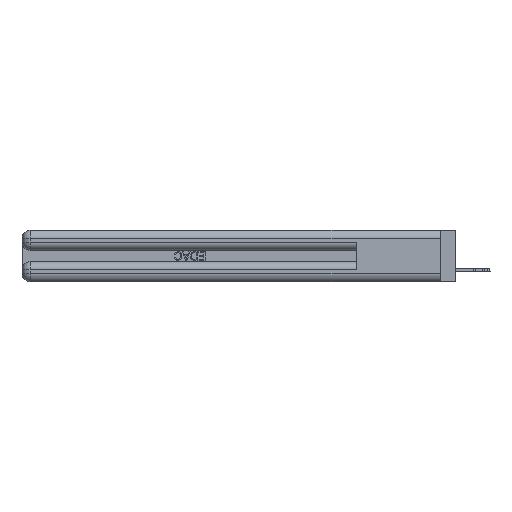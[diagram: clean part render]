
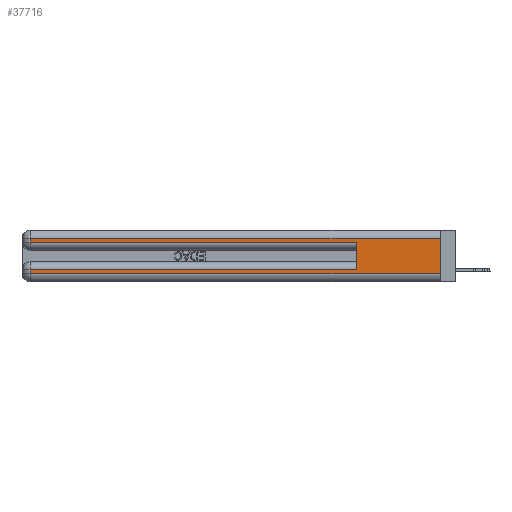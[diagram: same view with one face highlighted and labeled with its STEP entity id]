
A CAD part, left-side view. The second image highlights one B-rep face of the part: STEP entity #37716.
In plain terms, the highlighted planar face has unit normal (-1, 0, 0).
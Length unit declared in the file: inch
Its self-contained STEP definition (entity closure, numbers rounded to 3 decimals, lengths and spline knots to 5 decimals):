
#146 = ORIENTED_EDGE ( 'NONE', *, *, #33059, .T. ) ;
#435 = LINE ( 'NONE', #4650, #18090 ) ;
#865 = VECTOR ( 'NONE', #20401, 39.37008 ) ;
#1054 = FACE_OUTER_BOUND ( 'NONE', #14440, .T. ) ;
#1410 = VECTOR ( 'NONE', #2643, 39.37008 ) ;
#2643 = DIRECTION ( 'NONE',  ( 0., -1., 0. ) ) ;
#2742 = CARTESIAN_POINT ( 'NONE',  ( 0., 2.94, 0.37 ) ) ;
#2978 = EDGE_CURVE ( 'NONE', #9925, #3714, #24033, .T. ) ;
#3238 = LINE ( 'NONE', #29658, #37325 ) ;
#3714 = VERTEX_POINT ( 'NONE', #30575 ) ;
#3871 = VERTEX_POINT ( 'NONE', #29867 ) ;
#4545 = DIRECTION ( 'NONE',  ( 0., 0., -1. ) ) ;
#4615 = ORIENTED_EDGE ( 'NONE', *, *, #8156, .T. ) ;
#4650 = CARTESIAN_POINT ( 'NONE',  ( 0., 2.94, 0.37 ) ) ;
#4687 = CARTESIAN_POINT ( 'NONE',  ( 0., 0., 0.37 ) ) ;
#6514 = LINE ( 'NONE', #2742, #865 ) ;
#7656 = DIRECTION ( 'NONE',  ( 1., 0., 0. ) ) ;
#8156 = EDGE_CURVE ( 'NONE', #44690, #15455, #9622, .T. ) ;
#8501 = CARTESIAN_POINT ( 'NONE',  ( 0., 2.94, 0.285 ) ) ;
#9070 = VECTOR ( 'NONE', #27613, 39.37008 ) ;
#9185 = LINE ( 'NONE', #31111, #26742 ) ;
#9622 = LINE ( 'NONE', #34225, #9070 ) ;
#9773 = CARTESIAN_POINT ( 'NONE',  ( 0., 2.94, 0.31 ) ) ;
#9925 = VERTEX_POINT ( 'NONE', #41278 ) ;
#10658 = LINE ( 'NONE', #4687, #17779 ) ;
#10838 = ORIENTED_EDGE ( 'NONE', *, *, #19768, .T. ) ;
#11534 = VERTEX_POINT ( 'NONE', #9773 ) ;
#11912 = VERTEX_POINT ( 'NONE', #22294 ) ;
#13149 = ORIENTED_EDGE ( 'NONE', *, *, #36510, .F. ) ;
#14440 = EDGE_LOOP ( 'NONE', ( #13149, #28831, #29633, #146, #44325, #10838, #34735, #4615 ) ) ;
#15455 = VERTEX_POINT ( 'NONE', #20627 ) ;
#15961 = VERTEX_POINT ( 'NONE', #8501 ) ;
#17153 = DIRECTION ( 'NONE',  ( 0., 1., 0. ) ) ;
#17544 = LINE ( 'NONE', #30440, #1410 ) ;
#17552 = DIRECTION ( 'NONE',  ( 0., 0., 1. ) ) ;
#17779 = VECTOR ( 'NONE', #33285, 39.37008 ) ;
#18090 = VECTOR ( 'NONE', #43062, 39.37008 ) ;
#19768 = EDGE_CURVE ( 'NONE', #9925, #11912, #9185, .T. ) ;
#20401 = DIRECTION ( 'NONE',  ( 0., 0., -1. ) ) ;
#20627 = CARTESIAN_POINT ( 'NONE',  ( 0., 0., 0.06 ) ) ;
#21405 = EDGE_CURVE ( 'NONE', #3871, #11534, #3238, .T. ) ;
#22294 = CARTESIAN_POINT ( 'NONE',  ( 0., 2.94, 0.085 ) ) ;
#24033 = LINE ( 'NONE', #35057, #38911 ) ;
#24097 = CARTESIAN_POINT ( 'NONE',  ( 0., 2.94, 0.06 ) ) ;
#26742 = VECTOR ( 'NONE', #17153, 39.37008 ) ;
#27613 = DIRECTION ( 'NONE',  ( 0., -1., 0. ) ) ;
#28831 = ORIENTED_EDGE ( 'NONE', *, *, #21405, .T. ) ;
#29125 = CARTESIAN_POINT ( 'NONE',  ( 0., 0., 0.37 ) ) ;
#29633 = ORIENTED_EDGE ( 'NONE', *, *, #33791, .T. ) ;
#29658 = CARTESIAN_POINT ( 'NONE',  ( 0., 0., 0.31 ) ) ;
#29867 = CARTESIAN_POINT ( 'NONE',  ( 0., 0., 0.31 ) ) ;
#30440 = CARTESIAN_POINT ( 'NONE',  ( 0., 0., 0.285 ) ) ;
#30575 = CARTESIAN_POINT ( 'NONE',  ( 0., 0.6, 0.285 ) ) ;
#31111 = CARTESIAN_POINT ( 'NONE',  ( 0., 0., 0.085 ) ) ;
#33059 = EDGE_CURVE ( 'NONE', #15961, #3714, #17544, .T. ) ;
#33285 = DIRECTION ( 'NONE',  ( 0., 0., -1. ) ) ;
#33791 = EDGE_CURVE ( 'NONE', #11534, #15961, #6514, .T. ) ;
#34225 = CARTESIAN_POINT ( 'NONE',  ( 0., 0., 0.06 ) ) ;
#34735 = ORIENTED_EDGE ( 'NONE', *, *, #38486, .T. ) ;
#35057 = CARTESIAN_POINT ( 'NONE',  ( 0., 0.6, 0.145 ) ) ;
#36510 = EDGE_CURVE ( 'NONE', #3871, #15455, #10658, .T. ) ;
#37325 = VECTOR ( 'NONE', #40462, 39.37008 ) ;
#37716 = ADVANCED_FACE ( 'NONE', ( #1054 ), #45171, .F. ) ;
#38486 = EDGE_CURVE ( 'NONE', #11912, #44690, #435, .T. ) ;
#38911 = VECTOR ( 'NONE', #17552, 39.37008 ) ;
#40462 = DIRECTION ( 'NONE',  ( 0., 1., 0. ) ) ;
#40731 = AXIS2_PLACEMENT_3D ( 'NONE', #29125, #7656, #4545 ) ;
#41278 = CARTESIAN_POINT ( 'NONE',  ( 0., 0.6, 0.085 ) ) ;
#43062 = DIRECTION ( 'NONE',  ( 0., 0., -1. ) ) ;
#44325 = ORIENTED_EDGE ( 'NONE', *, *, #2978, .F. ) ;
#44690 = VERTEX_POINT ( 'NONE', #24097 ) ;
#45171 = PLANE ( 'NONE',  #40731 ) ;
